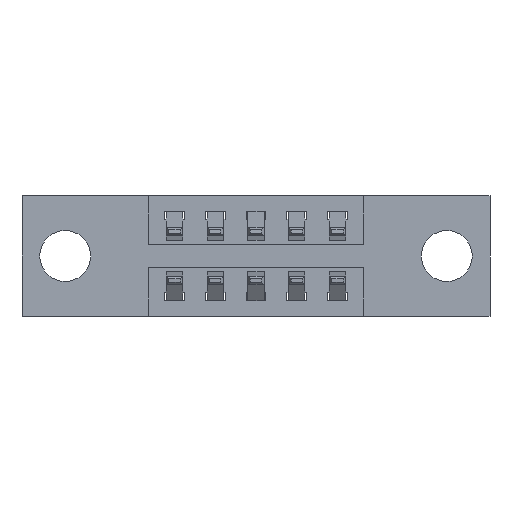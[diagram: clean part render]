
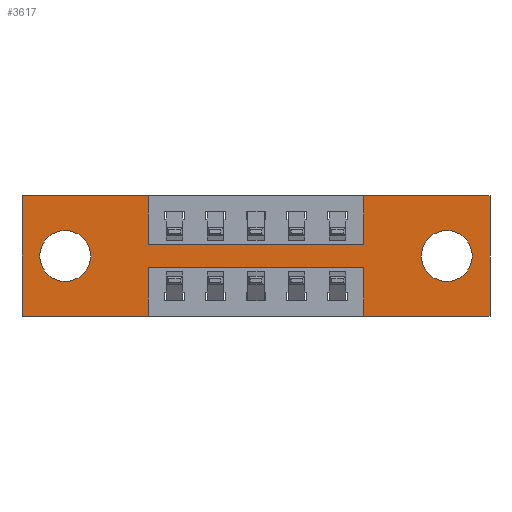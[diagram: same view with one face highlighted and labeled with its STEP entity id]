
A CAD part, front view. The second image highlights one B-rep face of the part: STEP entity #3617.
In plain terms, the highlighted planar face has unit normal (0, -1, 0).
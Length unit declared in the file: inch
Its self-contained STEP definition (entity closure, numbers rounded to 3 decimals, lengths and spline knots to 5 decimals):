
#29 = VERTEX_POINT ( 'NONE', #1852 ) ;
#323 = VECTOR ( 'NONE', #7424, 39.37008 ) ;
#358 = VECTOR ( 'NONE', #1928, 39.37008 ) ;
#369 = LINE ( 'NONE', #4581, #323 ) ;
#380 = EDGE_LOOP ( 'NONE', ( #7448, #7885, #1223, #5450, #8001, #7091, #6889, #8235, #8281, #6162, #2041, #5475 ) ) ;
#388 = VECTOR ( 'NONE', #2942, 39.37008 ) ;
#405 = LINE ( 'NONE', #7822, #358 ) ;
#416 = VECTOR ( 'NONE', #6491, 39.37008 ) ;
#422 = LINE ( 'NONE', #557, #416 ) ;
#429 = LINE ( 'NONE', #6714, #449 ) ;
#442 = VECTOR ( 'NONE', #8114, 39.37008 ) ;
#449 = VECTOR ( 'NONE', #5912, 39.37008 ) ;
#457 = LINE ( 'NONE', #6429, #388 ) ;
#470 = CIRCLE ( 'NONE', #906, 0.078 ) ;
#485 = LINE ( 'NONE', #6727, #442 ) ;
#528 = CIRCLE ( 'NONE', #1023, 0.078 ) ;
#538 = VECTOR ( 'NONE', #6680, 39.37008 ) ;
#557 = CARTESIAN_POINT ( 'NONE',  ( 0.3875, 0., -0.22 ) ) ;
#570 = VECTOR ( 'NONE', #7791, 39.37008 ) ;
#581 = DIRECTION ( 'NONE',  ( 1., 0., 0. ) ) ;
#592 = LINE ( 'NONE', #7685, #538 ) ;
#623 = LINE ( 'NONE', #7558, #570 ) ;
#648 = VECTOR ( 'NONE', #8063, 39.37008 ) ;
#652 = DIRECTION ( 'NONE',  ( 0., 0., 1. ) ) ;
#685 = LINE ( 'NONE', #1716, #648 ) ;
#699 = VERTEX_POINT ( 'NONE', #6583 ) ;
#721 = VECTOR ( 'NONE', #7402, 39.37008 ) ;
#743 = CARTESIAN_POINT ( 'NONE',  ( 0.1325, 0., -0.263 ) ) ;
#760 = LINE ( 'NONE', #7590, #721 ) ;
#774 = VECTOR ( 'NONE', #652, 39.37008 ) ;
#809 = EDGE_CURVE ( 'NONE', #6081, #3705, #844, .T. ) ;
#827 = EDGE_CURVE ( 'NONE', #8093, #4769, #760, .T. ) ;
#843 = EDGE_CURVE ( 'NONE', #4769, #5859, #685, .T. ) ;
#844 = LINE ( 'NONE', #1189, #774 ) ;
#862 = EDGE_CURVE ( 'NONE', #3628, #6081, #623, .T. ) ;
#865 = EDGE_CURVE ( 'NONE', #3705, #2537, #592, .T. ) ;
#882 = CARTESIAN_POINT ( 'NONE',  ( 0., 0., 0. ) ) ;
#894 = EDGE_CURVE ( 'NONE', #6202, #3030, #528, .T. ) ;
#897 = EDGE_CURVE ( 'NONE', #5582, #5948, #470, .T. ) ;
#898 = EDGE_CURVE ( 'NONE', #29, #3628, #485, .T. ) ;
#906 = AXIS2_PLACEMENT_3D ( 'NONE', #7326, #3926, #7617 ) ;
#911 = EDGE_CURVE ( 'NONE', #699, #29, #422, .T. ) ;
#913 = EDGE_CURVE ( 'NONE', #5859, #699, #429, .T. ) ;
#917 = EDGE_CURVE ( 'NONE', #4634, #7875, #457, .T. ) ;
#929 = EDGE_CURVE ( 'NONE', #3383, #4634, #405, .T. ) ;
#931 = EDGE_CURVE ( 'NONE', #2537, #3383, #369, .T. ) ;
#1023 = AXIS2_PLACEMENT_3D ( 'NONE', #4478, #4469, #6760 ) ;
#1189 = CARTESIAN_POINT ( 'NONE',  ( 0., 0., 0. ) ) ;
#1223 = ORIENTED_EDGE ( 'NONE', *, *, #913, .F. ) ;
#1716 = CARTESIAN_POINT ( 'NONE',  ( 0., 0., -0.37 ) ) ;
#1852 = CARTESIAN_POINT ( 'NONE',  ( 0.3875, 0., -0.22 ) ) ;
#1928 = DIRECTION ( 'NONE',  ( 1., 0., 0. ) ) ;
#2009 = CARTESIAN_POINT ( 'NONE',  ( 0.1325, 0., -0.107 ) ) ;
#2041 = ORIENTED_EDGE ( 'NONE', *, *, #809, .F. ) ;
#2119 = DIRECTION ( 'NONE',  ( 0., 0., -1. ) ) ;
#2157 = ORIENTED_EDGE ( 'NONE', *, *, #3381, .T. ) ;
#2275 = AXIS2_PLACEMENT_3D ( 'NONE', #2496, #2549, #2119 ) ;
#2496 = CARTESIAN_POINT ( 'NONE',  ( 1.3025, 0., -0.185 ) ) ;
#2537 = VERTEX_POINT ( 'NONE', #5968 ) ;
#2549 = DIRECTION ( 'NONE',  ( 0., 1., 0. ) ) ;
#2724 = ORIENTED_EDGE ( 'NONE', *, *, #894, .T. ) ;
#2942 = DIRECTION ( 'NONE',  ( 0., 0., 1. ) ) ;
#3030 = VERTEX_POINT ( 'NONE', #7060 ) ;
#3371 = CARTESIAN_POINT ( 'NONE',  ( 0., 0., 0. ) ) ;
#3381 = EDGE_CURVE ( 'NONE', #3030, #6202, #5028, .T. ) ;
#3383 = VERTEX_POINT ( 'NONE', #4406 ) ;
#3617 = ADVANCED_FACE ( 'NONE', ( #4297, #4245, #4172 ), #5937, .T. ) ;
#3628 = VERTEX_POINT ( 'NONE', #5989 ) ;
#3705 = VERTEX_POINT ( 'NONE', #3371 ) ;
#3745 = AXIS2_PLACEMENT_3D ( 'NONE', #7106, #6393, #5522 ) ;
#3926 = DIRECTION ( 'NONE',  ( 0., 1., 0. ) ) ;
#3932 = CARTESIAN_POINT ( 'NONE',  ( 1.0475, 0., -0.37 ) ) ;
#3989 = CIRCLE ( 'NONE', #7020, 0.078 ) ;
#4161 = EDGE_CURVE ( 'NONE', #7875, #8093, #4257, .T. ) ;
#4172 = FACE_OUTER_BOUND ( 'NONE', #380, .T. ) ;
#4207 = ORIENTED_EDGE ( 'NONE', *, *, #897, .T. ) ;
#4233 = EDGE_CURVE ( 'NONE', #5948, #5582, #3989, .T. ) ;
#4245 = FACE_BOUND ( 'NONE', #5221, .T. ) ;
#4252 = VECTOR ( 'NONE', #581, 39.37008 ) ;
#4257 = LINE ( 'NONE', #882, #4252 ) ;
#4297 = FACE_BOUND ( 'NONE', #5205, .T. ) ;
#4406 = CARTESIAN_POINT ( 'NONE',  ( 0.3875, 0., -0.15 ) ) ;
#4469 = DIRECTION ( 'NONE',  ( 0., 1., 0. ) ) ;
#4478 = CARTESIAN_POINT ( 'NONE',  ( 1.3025, 0., -0.185 ) ) ;
#4581 = CARTESIAN_POINT ( 'NONE',  ( 0.3875, 0., 0. ) ) ;
#4634 = VERTEX_POINT ( 'NONE', #8273 ) ;
#4769 = VERTEX_POINT ( 'NONE', #7278 ) ;
#4903 = ORIENTED_EDGE ( 'NONE', *, *, #4233, .T. ) ;
#5028 = CIRCLE ( 'NONE', #2275, 0.078 ) ;
#5205 = EDGE_LOOP ( 'NONE', ( #2724, #2157 ) ) ;
#5221 = EDGE_LOOP ( 'NONE', ( #4207, #4903 ) ) ;
#5441 = CARTESIAN_POINT ( 'NONE',  ( 0., 0., -0.37 ) ) ;
#5450 = ORIENTED_EDGE ( 'NONE', *, *, #843, .F. ) ;
#5475 = ORIENTED_EDGE ( 'NONE', *, *, #862, .F. ) ;
#5522 = DIRECTION ( 'NONE',  ( 0., 0., -1. ) ) ;
#5534 = CARTESIAN_POINT ( 'NONE',  ( 1.3025, 0., -0.107 ) ) ;
#5582 = VERTEX_POINT ( 'NONE', #2009 ) ;
#5859 = VERTEX_POINT ( 'NONE', #3932 ) ;
#5912 = DIRECTION ( 'NONE',  ( 0., 0., 1. ) ) ;
#5937 = PLANE ( 'NONE',  #3745 ) ;
#5948 = VERTEX_POINT ( 'NONE', #743 ) ;
#5968 = CARTESIAN_POINT ( 'NONE',  ( 0.3875, 0., 0. ) ) ;
#5989 = CARTESIAN_POINT ( 'NONE',  ( 0.3875, 0., -0.37 ) ) ;
#6081 = VERTEX_POINT ( 'NONE', #5441 ) ;
#6162 = ORIENTED_EDGE ( 'NONE', *, *, #865, .F. ) ;
#6202 = VERTEX_POINT ( 'NONE', #5534 ) ;
#6393 = DIRECTION ( 'NONE',  ( 0., -1., 0. ) ) ;
#6429 = CARTESIAN_POINT ( 'NONE',  ( 1.0475, 0., 0. ) ) ;
#6491 = DIRECTION ( 'NONE',  ( -1., 0., 0. ) ) ;
#6583 = CARTESIAN_POINT ( 'NONE',  ( 1.0475, 0., -0.22 ) ) ;
#6680 = DIRECTION ( 'NONE',  ( 1., 0., 0. ) ) ;
#6714 = CARTESIAN_POINT ( 'NONE',  ( 1.0475, 0., -0.37 ) ) ;
#6727 = CARTESIAN_POINT ( 'NONE',  ( 0.3875, 0., -0.37 ) ) ;
#6760 = DIRECTION ( 'NONE',  ( 0., 0., -1. ) ) ;
#6889 = ORIENTED_EDGE ( 'NONE', *, *, #917, .F. ) ;
#7020 = AXIS2_PLACEMENT_3D ( 'NONE', #8228, #7919, #7770 ) ;
#7060 = CARTESIAN_POINT ( 'NONE',  ( 1.3025, 0., -0.263 ) ) ;
#7091 = ORIENTED_EDGE ( 'NONE', *, *, #4161, .F. ) ;
#7106 = CARTESIAN_POINT ( 'NONE',  ( 0., 0., -0.37 ) ) ;
#7278 = CARTESIAN_POINT ( 'NONE',  ( 1.435, 0., -0.37 ) ) ;
#7326 = CARTESIAN_POINT ( 'NONE',  ( 0.1325, 0., -0.185 ) ) ;
#7338 = CARTESIAN_POINT ( 'NONE',  ( 1.435, 0., 0. ) ) ;
#7402 = DIRECTION ( 'NONE',  ( 0., 0., -1. ) ) ;
#7424 = DIRECTION ( 'NONE',  ( 0., 0., -1. ) ) ;
#7448 = ORIENTED_EDGE ( 'NONE', *, *, #898, .F. ) ;
#7558 = CARTESIAN_POINT ( 'NONE',  ( 0., 0., -0.37 ) ) ;
#7590 = CARTESIAN_POINT ( 'NONE',  ( 1.435, 0., 0. ) ) ;
#7617 = DIRECTION ( 'NONE',  ( 0., 0., 1. ) ) ;
#7685 = CARTESIAN_POINT ( 'NONE',  ( 0., 0., 0. ) ) ;
#7770 = DIRECTION ( 'NONE',  ( 0., 0., 1. ) ) ;
#7791 = DIRECTION ( 'NONE',  ( -1., 0., 0. ) ) ;
#7822 = CARTESIAN_POINT ( 'NONE',  ( 0.3875, 0., -0.15 ) ) ;
#7875 = VERTEX_POINT ( 'NONE', #8097 ) ;
#7885 = ORIENTED_EDGE ( 'NONE', *, *, #911, .F. ) ;
#7919 = DIRECTION ( 'NONE',  ( 0., 1., 0. ) ) ;
#8001 = ORIENTED_EDGE ( 'NONE', *, *, #827, .F. ) ;
#8063 = DIRECTION ( 'NONE',  ( -1., 0., 0. ) ) ;
#8093 = VERTEX_POINT ( 'NONE', #7338 ) ;
#8097 = CARTESIAN_POINT ( 'NONE',  ( 1.0475, 0., 0. ) ) ;
#8114 = DIRECTION ( 'NONE',  ( 0., 0., -1. ) ) ;
#8228 = CARTESIAN_POINT ( 'NONE',  ( 0.1325, 0., -0.185 ) ) ;
#8235 = ORIENTED_EDGE ( 'NONE', *, *, #929, .F. ) ;
#8273 = CARTESIAN_POINT ( 'NONE',  ( 1.0475, 0., -0.15 ) ) ;
#8281 = ORIENTED_EDGE ( 'NONE', *, *, #931, .F. ) ;
